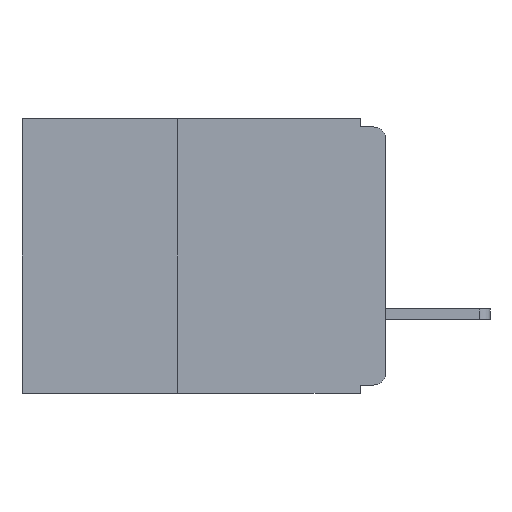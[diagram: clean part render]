
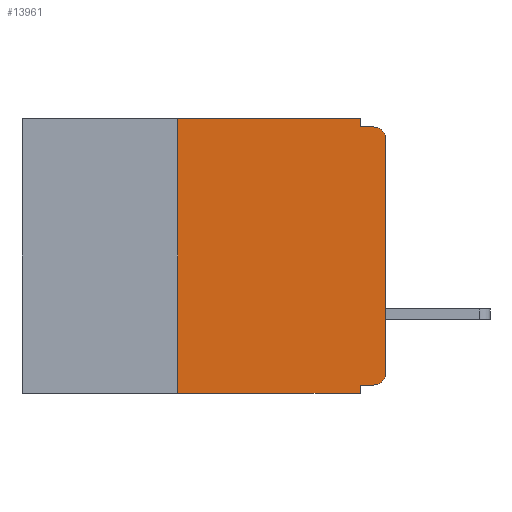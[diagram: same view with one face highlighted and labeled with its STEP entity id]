
A CAD part, left-side view. The second image highlights one B-rep face of the part: STEP entity #13961.
In plain terms, the highlighted planar face has unit normal (-1, 0, 0).
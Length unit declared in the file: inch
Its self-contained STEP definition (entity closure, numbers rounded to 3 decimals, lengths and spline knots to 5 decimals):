
#325 = CARTESIAN_POINT ( 'NONE',  ( 0., 0.25, -0.33 ) ) ;
#725 = DIRECTION ( 'NONE',  ( 0., 0., 1. ) ) ;
#873 = CARTESIAN_POINT ( 'NONE',  ( 0., 0.031, -0.33 ) ) ;
#1394 = LINE ( 'NONE', #14927, #1430 ) ;
#1430 = VECTOR ( 'NONE', #14903, 39.37008 ) ;
#1732 = CARTESIAN_POINT ( 'NONE',  ( 0., 0.031, 0. ) ) ;
#2874 = VECTOR ( 'NONE', #725, 39.37008 ) ;
#2971 = ORIENTED_EDGE ( 'NONE', *, *, #15220, .F. ) ;
#3022 = LINE ( 'NONE', #325, #2874 ) ;
#3236 = CARTESIAN_POINT ( 'NONE',  ( 0., 0.015, -0.32 ) ) ;
#3617 = EDGE_CURVE ( 'NONE', #3641, #14615, #6226, .T. ) ;
#3641 = VERTEX_POINT ( 'NONE', #14558 ) ;
#3979 = ORIENTED_EDGE ( 'NONE', *, *, #3617, .T. ) ;
#4030 = ORIENTED_EDGE ( 'NONE', *, *, #14031, .T. ) ;
#4179 = EDGE_LOOP ( 'NONE', ( #3979, #4030, #6161, #8195, #9396, #2971, #4335, #7657, #9329, #12876 ) ) ;
#4335 = ORIENTED_EDGE ( 'NONE', *, *, #15576, .T. ) ;
#4428 = VERTEX_POINT ( 'NONE', #873 ) ;
#4770 = CARTESIAN_POINT ( 'NONE',  ( 0., 0.015, -0.01 ) ) ;
#5405 = CARTESIAN_POINT ( 'NONE',  ( 0., 0.25, 0. ) ) ;
#5413 = VECTOR ( 'NONE', #17897, 39.37008 ) ;
#5457 = LINE ( 'NONE', #18015, #5413 ) ;
#5559 = VERTEX_POINT ( 'NONE', #3236 ) ;
#6123 = VECTOR ( 'NONE', #14897, 39.37008 ) ;
#6161 = ORIENTED_EDGE ( 'NONE', *, *, #17103, .F. ) ;
#6226 = LINE ( 'NONE', #15816, #6123 ) ;
#6483 = DIRECTION ( 'NONE',  ( 0., 0., -1. ) ) ;
#6545 = DIRECTION ( 'NONE',  ( -1., 0., 0. ) ) ;
#6593 = CARTESIAN_POINT ( 'NONE',  ( 0., 0.015, -0.025 ) ) ;
#7035 = AXIS2_PLACEMENT_3D ( 'NONE', #8034, #7904, #7881 ) ;
#7192 = CARTESIAN_POINT ( 'NONE',  ( 0., 0., -0.025 ) ) ;
#7573 = DIRECTION ( 'NONE',  ( 0., 0., -1. ) ) ;
#7578 = DIRECTION ( 'NONE',  ( -1., 0., 0. ) ) ;
#7613 = CARTESIAN_POINT ( 'NONE',  ( 0., 0.015, -0.305 ) ) ;
#7657 = ORIENTED_EDGE ( 'NONE', *, *, #16004, .F. ) ;
#7784 = VERTEX_POINT ( 'NONE', #12493 ) ;
#7881 = DIRECTION ( 'NONE',  ( 0., 0., -1. ) ) ;
#7904 = DIRECTION ( 'NONE',  ( 1., 0., 0. ) ) ;
#8034 = CARTESIAN_POINT ( 'NONE',  ( 0., 0.437, 0. ) ) ;
#8195 = ORIENTED_EDGE ( 'NONE', *, *, #9637, .F. ) ;
#8208 = CIRCLE ( 'NONE', #10091, 0.015 ) ;
#8230 = CARTESIAN_POINT ( 'NONE',  ( 0., 0.031, -0.32 ) ) ;
#8247 = PLANE ( 'NONE',  #7035 ) ;
#8421 = FACE_OUTER_BOUND ( 'NONE', #4179, .T. ) ;
#9176 = AXIS2_PLACEMENT_3D ( 'NONE', #7613, #7578, #7573 ) ;
#9329 = ORIENTED_EDGE ( 'NONE', *, *, #14682, .F. ) ;
#9396 = ORIENTED_EDGE ( 'NONE', *, *, #12153, .F. ) ;
#9556 = VERTEX_POINT ( 'NONE', #16188 ) ;
#9637 = EDGE_CURVE ( 'NONE', #10087, #9556, #12456, .T. ) ;
#10087 = VERTEX_POINT ( 'NONE', #1732 ) ;
#10091 = AXIS2_PLACEMENT_3D ( 'NONE', #6593, #6545, #6483 ) ;
#10552 = VERTEX_POINT ( 'NONE', #4770 ) ;
#10743 = VERTEX_POINT ( 'NONE', #5405 ) ;
#11911 = VECTOR ( 'NONE', #17831, 39.37008 ) ;
#11923 = LINE ( 'NONE', #18075, #11911 ) ;
#12153 = EDGE_CURVE ( 'NONE', #10743, #10087, #14785, .T. ) ;
#12261 = VERTEX_POINT ( 'NONE', #8230 ) ;
#12452 = VECTOR ( 'NONE', #12779, 39.37008 ) ;
#12456 = LINE ( 'NONE', #13191, #12452 ) ;
#12493 = CARTESIAN_POINT ( 'NONE',  ( 0., 0.25, -0.33 ) ) ;
#12633 = CIRCLE ( 'NONE', #9176, 0.015 ) ;
#12779 = DIRECTION ( 'NONE',  ( 0., 0., -1. ) ) ;
#12838 = EDGE_CURVE ( 'NONE', #5559, #3641, #12633, .T. ) ;
#12876 = ORIENTED_EDGE ( 'NONE', *, *, #12838, .T. ) ;
#13191 = CARTESIAN_POINT ( 'NONE',  ( 0., 0.031, 0. ) ) ;
#13400 = DIRECTION ( 'NONE',  ( 0., -1., 0. ) ) ;
#13661 = CARTESIAN_POINT ( 'NONE',  ( 0., 0.437, 0. ) ) ;
#13961 = ADVANCED_FACE ( 'NONE', ( #8421 ), #8247, .F. ) ;
#14031 = EDGE_CURVE ( 'NONE', #14615, #10552, #8208, .T. ) ;
#14558 = CARTESIAN_POINT ( 'NONE',  ( 0., 0., -0.305 ) ) ;
#14615 = VERTEX_POINT ( 'NONE', #7192 ) ;
#14682 = EDGE_CURVE ( 'NONE', #5559, #12261, #5457, .T. ) ;
#14738 = VECTOR ( 'NONE', #13400, 39.37008 ) ;
#14750 = DIRECTION ( 'NONE',  ( 0., 0., -1. ) ) ;
#14785 = LINE ( 'NONE', #13661, #14738 ) ;
#14897 = DIRECTION ( 'NONE',  ( 0., 0., 1. ) ) ;
#14903 = DIRECTION ( 'NONE',  ( 0., -1., 0. ) ) ;
#14927 = CARTESIAN_POINT ( 'NONE',  ( 0., 0.437, -0.33 ) ) ;
#15220 = EDGE_CURVE ( 'NONE', #7784, #10743, #3022, .T. ) ;
#15576 = EDGE_CURVE ( 'NONE', #7784, #4428, #1394, .T. ) ;
#15732 = CARTESIAN_POINT ( 'NONE',  ( 0., 0.031, -0.33 ) ) ;
#15816 = CARTESIAN_POINT ( 'NONE',  ( 0., 0., 0. ) ) ;
#16004 = EDGE_CURVE ( 'NONE', #12261, #4428, #16656, .T. ) ;
#16188 = CARTESIAN_POINT ( 'NONE',  ( 0., 0.031, -0.01 ) ) ;
#16405 = VECTOR ( 'NONE', #14750, 39.37008 ) ;
#16656 = LINE ( 'NONE', #15732, #16405 ) ;
#17103 = EDGE_CURVE ( 'NONE', #9556, #10552, #11923, .T. ) ;
#17831 = DIRECTION ( 'NONE',  ( 0., -1., 0. ) ) ;
#17897 = DIRECTION ( 'NONE',  ( 0., 1., 0. ) ) ;
#18015 = CARTESIAN_POINT ( 'NONE',  ( 0., 0., -0.32 ) ) ;
#18075 = CARTESIAN_POINT ( 'NONE',  ( 0., 0., -0.01 ) ) ;
